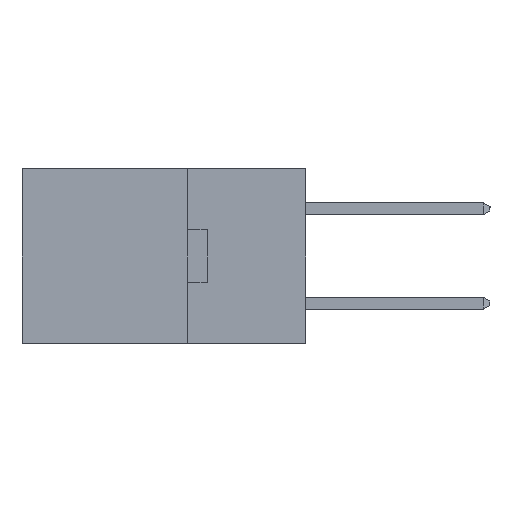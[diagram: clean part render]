
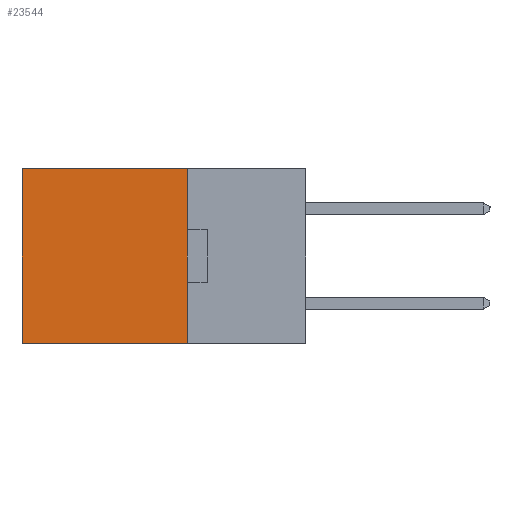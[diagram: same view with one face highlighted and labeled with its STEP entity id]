
A CAD part, left-side view. The second image highlights one B-rep face of the part: STEP entity #23544.
In plain terms, the highlighted planar face has unit normal (-1, 0, 0).
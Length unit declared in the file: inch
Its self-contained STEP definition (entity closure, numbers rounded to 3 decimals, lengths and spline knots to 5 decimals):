
#126 = DIRECTION ( 'NONE',  ( 0., 0., -1. ) ) ;
#821 = LINE ( 'NONE', #20243, #21468 ) ;
#1678 = VERTEX_POINT ( 'NONE', #9868 ) ;
#3070 = ORIENTED_EDGE ( 'NONE', *, *, #28125, .T. ) ;
#3894 = VECTOR ( 'NONE', #13624, 39.37008 ) ;
#3957 = EDGE_CURVE ( 'NONE', #1678, #22983, #821, .T. ) ;
#4913 = CARTESIAN_POINT ( 'NONE',  ( 0.2615, 0.25, 0. ) ) ;
#5363 = EDGE_LOOP ( 'NONE', ( #9547, #8974, #7486, #3070 ) ) ;
#6375 = CARTESIAN_POINT ( 'NONE',  ( 0.2615, 0.6, 0. ) ) ;
#7486 = ORIENTED_EDGE ( 'NONE', *, *, #3957, .F. ) ;
#8179 = CARTESIAN_POINT ( 'NONE',  ( 0.2615, 0.6, -0.37 ) ) ;
#8717 = CARTESIAN_POINT ( 'NONE',  ( 0.2615, 0.25, -0.37 ) ) ;
#8974 = ORIENTED_EDGE ( 'NONE', *, *, #17824, .F. ) ;
#9529 = CARTESIAN_POINT ( 'NONE',  ( 0.2615, 0.25, -0.37 ) ) ;
#9530 = DIRECTION ( 'NONE',  ( 0., 0., -1. ) ) ;
#9547 = ORIENTED_EDGE ( 'NONE', *, *, #20951, .T. ) ;
#9868 = CARTESIAN_POINT ( 'NONE',  ( 0.2615, 0.25, 0. ) ) ;
#13149 = LINE ( 'NONE', #8179, #16456 ) ;
#13624 = DIRECTION ( 'NONE',  ( 0., 1., 0. ) ) ;
#13698 = DIRECTION ( 'NONE',  ( 1., 0., 0. ) ) ;
#15440 = LINE ( 'NONE', #22025, #26979 ) ;
#16456 = VECTOR ( 'NONE', #126, 39.37008 ) ;
#16575 = VERTEX_POINT ( 'NONE', #24267 ) ;
#17098 = VERTEX_POINT ( 'NONE', #6375 ) ;
#17824 = EDGE_CURVE ( 'NONE', #22983, #16575, #15440, .T. ) ;
#18093 = DIRECTION ( 'NONE',  ( 0., 0., -1. ) ) ;
#19585 = DIRECTION ( 'NONE',  ( 0., 1., 0. ) ) ;
#20243 = CARTESIAN_POINT ( 'NONE',  ( 0.2615, 0.25, -0.37 ) ) ;
#20951 = EDGE_CURVE ( 'NONE', #17098, #16575, #13149, .T. ) ;
#21468 = VECTOR ( 'NONE', #9530, 39.37008 ) ;
#22025 = CARTESIAN_POINT ( 'NONE',  ( 0.2615, 0.25, -0.37 ) ) ;
#22962 = AXIS2_PLACEMENT_3D ( 'NONE', #9529, #13698, #18093 ) ;
#22983 = VERTEX_POINT ( 'NONE', #8717 ) ;
#23544 = ADVANCED_FACE ( 'NONE', ( #26710 ), #24555, .F. ) ;
#24267 = CARTESIAN_POINT ( 'NONE',  ( 0.2615, 0.6, -0.37 ) ) ;
#24479 = LINE ( 'NONE', #4913, #3894 ) ;
#24555 = PLANE ( 'NONE',  #22962 ) ;
#26710 = FACE_OUTER_BOUND ( 'NONE', #5363, .T. ) ;
#26979 = VECTOR ( 'NONE', #19585, 39.37008 ) ;
#28125 = EDGE_CURVE ( 'NONE', #1678, #17098, #24479, .T. ) ;
